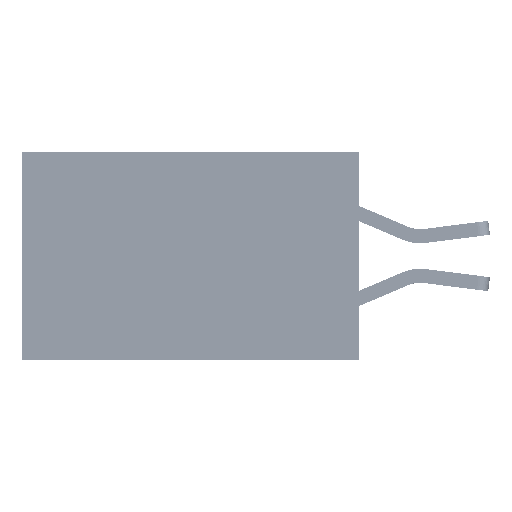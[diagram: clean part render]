
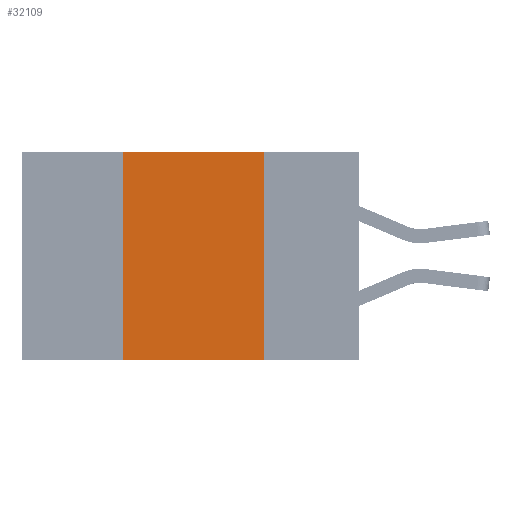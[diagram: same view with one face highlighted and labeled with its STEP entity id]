
A CAD part, left-side view. The second image highlights one B-rep face of the part: STEP entity #32109.
In plain terms, the highlighted planar face has unit normal (-1, 0, 0).
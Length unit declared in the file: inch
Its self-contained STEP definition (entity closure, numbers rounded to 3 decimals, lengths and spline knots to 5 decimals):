
#1918 = DIRECTION ( 'NONE',  ( 0., 0., -1. ) ) ;
#2480 = VERTEX_POINT ( 'NONE', #27982 ) ;
#2501 = DIRECTION ( 'NONE',  ( 0., 0., 1. ) ) ;
#3593 = FACE_OUTER_BOUND ( 'NONE', #22495, .T. ) ;
#4471 = DIRECTION ( 'NONE',  ( 0., 0., -1. ) ) ;
#7492 = VECTOR ( 'NONE', #2501, 39.37008 ) ;
#8411 = DIRECTION ( 'NONE',  ( 0., -1., 0. ) ) ;
#8667 = DIRECTION ( 'NONE',  ( 0., -1., 0. ) ) ;
#8834 = CARTESIAN_POINT ( 'NONE',  ( 0., 0.6, 0. ) ) ;
#9678 = ORIENTED_EDGE ( 'NONE', *, *, #11483, .F. ) ;
#9913 = LINE ( 'NONE', #15889, #13401 ) ;
#10349 = CARTESIAN_POINT ( 'NONE',  ( 0., 0.42, 0. ) ) ;
#11468 = CARTESIAN_POINT ( 'NONE',  ( 0., 0.17, -0.37 ) ) ;
#11483 = EDGE_CURVE ( 'NONE', #2480, #44195, #20297, .T. ) ;
#13313 = CARTESIAN_POINT ( 'NONE',  ( 0., 0.17, 0. ) ) ;
#13401 = VECTOR ( 'NONE', #8411, 39.37008 ) ;
#15585 = VECTOR ( 'NONE', #1918, 39.37008 ) ;
#15889 = CARTESIAN_POINT ( 'NONE',  ( 0., 0.6, -0.37 ) ) ;
#16024 = EDGE_CURVE ( 'NONE', #23395, #2480, #32561, .T. ) ;
#19618 = AXIS2_PLACEMENT_3D ( 'NONE', #19632, #45821, #4471 ) ;
#19632 = CARTESIAN_POINT ( 'NONE',  ( 0., 0.6, 0. ) ) ;
#20297 = LINE ( 'NONE', #13313, #15585 ) ;
#21478 = VECTOR ( 'NONE', #8667, 39.37008 ) ;
#22495 = EDGE_LOOP ( 'NONE', ( #9678, #26982, #48280, #39303 ) ) ;
#23395 = VERTEX_POINT ( 'NONE', #33040 ) ;
#23730 = EDGE_CURVE ( 'NONE', #43233, #23395, #33764, .T. ) ;
#26982 = ORIENTED_EDGE ( 'NONE', *, *, #16024, .F. ) ;
#27142 = EDGE_CURVE ( 'NONE', #43233, #44195, #9913, .T. ) ;
#27499 = PLANE ( 'NONE',  #19618 ) ;
#27982 = CARTESIAN_POINT ( 'NONE',  ( 0., 0.17, 0. ) ) ;
#32109 = ADVANCED_FACE ( 'NONE', ( #3593 ), #27499, .F. ) ;
#32561 = LINE ( 'NONE', #8834, #21478 ) ;
#33040 = CARTESIAN_POINT ( 'NONE',  ( 0., 0.42, 0. ) ) ;
#33764 = LINE ( 'NONE', #10349, #7492 ) ;
#39303 = ORIENTED_EDGE ( 'NONE', *, *, #27142, .T. ) ;
#43233 = VERTEX_POINT ( 'NONE', #47567 ) ;
#44195 = VERTEX_POINT ( 'NONE', #11468 ) ;
#45821 = DIRECTION ( 'NONE',  ( 1., 0., 0. ) ) ;
#47567 = CARTESIAN_POINT ( 'NONE',  ( 0., 0.42, -0.37 ) ) ;
#48280 = ORIENTED_EDGE ( 'NONE', *, *, #23730, .F. ) ;
